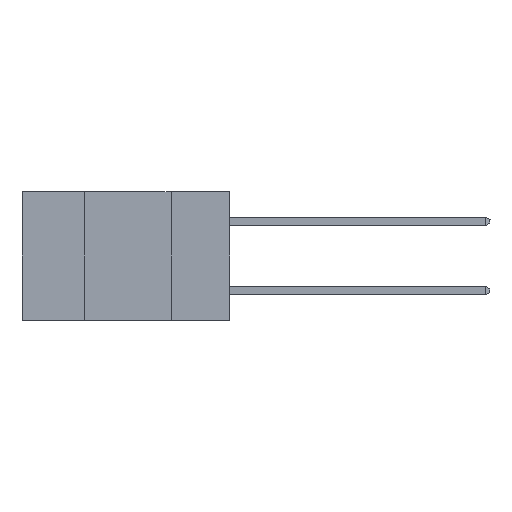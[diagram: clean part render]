
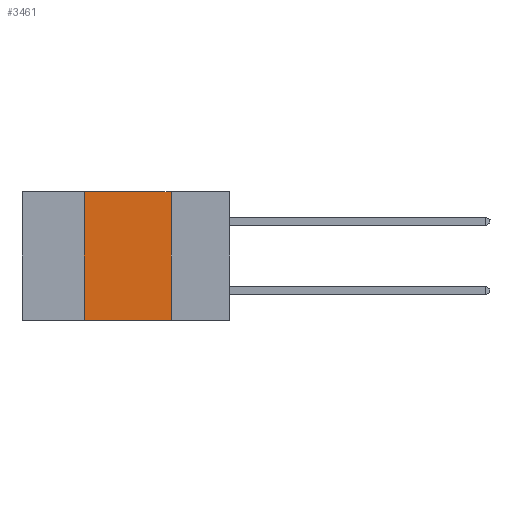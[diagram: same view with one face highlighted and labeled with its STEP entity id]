
A CAD part, left-side view. The second image highlights one B-rep face of the part: STEP entity #3461.
In plain terms, the highlighted planar face has unit normal (-1, 0, 0).
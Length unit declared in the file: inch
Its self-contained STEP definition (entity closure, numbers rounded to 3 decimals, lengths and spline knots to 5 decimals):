
#153 = CARTESIAN_POINT ( 'NONE',  ( 0., 0.17, -0.37 ) ) ;
#271 = DIRECTION ( 'NONE',  ( 0., 0., -1. ) ) ;
#1274 = EDGE_CURVE ( 'NONE', #13791, #14344, #12036, .T. ) ;
#1382 = FACE_OUTER_BOUND ( 'NONE', #9285, .T. ) ;
#2335 = DIRECTION ( 'NONE',  ( 0., -1., 0. ) ) ;
#3461 = ADVANCED_FACE ( 'NONE', ( #1382 ), #6351, .F. ) ;
#3529 = ORIENTED_EDGE ( 'NONE', *, *, #1274, .F. ) ;
#4554 = DIRECTION ( 'NONE',  ( 1., 0., 0. ) ) ;
#6351 = PLANE ( 'NONE',  #21138 ) ;
#7571 = LINE ( 'NONE', #23868, #23378 ) ;
#7751 = EDGE_CURVE ( 'NONE', #14344, #20612, #7571, .T. ) ;
#8056 = LINE ( 'NONE', #14474, #9948 ) ;
#9285 = EDGE_LOOP ( 'NONE', ( #13875, #3529, #11448, #18475 ) ) ;
#9948 = VECTOR ( 'NONE', #12006, 39.37008 ) ;
#10503 = CARTESIAN_POINT ( 'NONE',  ( 0., 0.6, 0. ) ) ;
#11448 = ORIENTED_EDGE ( 'NONE', *, *, #13153, .F. ) ;
#12006 = DIRECTION ( 'NONE',  ( 0., 0., 1. ) ) ;
#12036 = LINE ( 'NONE', #17709, #13574 ) ;
#13153 = EDGE_CURVE ( 'NONE', #13260, #13791, #8056, .T. ) ;
#13260 = VERTEX_POINT ( 'NONE', #22858 ) ;
#13574 = VECTOR ( 'NONE', #19741, 39.37008 ) ;
#13791 = VERTEX_POINT ( 'NONE', #21204 ) ;
#13875 = ORIENTED_EDGE ( 'NONE', *, *, #7751, .F. ) ;
#14344 = VERTEX_POINT ( 'NONE', #19740 ) ;
#14474 = CARTESIAN_POINT ( 'NONE',  ( 0., 0.42, 0. ) ) ;
#17122 = VECTOR ( 'NONE', #2335, 39.37008 ) ;
#17709 = CARTESIAN_POINT ( 'NONE',  ( 0., 0.6, 0. ) ) ;
#17733 = LINE ( 'NONE', #24817, #17122 ) ;
#18475 = ORIENTED_EDGE ( 'NONE', *, *, #24310, .T. ) ;
#19740 = CARTESIAN_POINT ( 'NONE',  ( 0., 0.17, 0. ) ) ;
#19741 = DIRECTION ( 'NONE',  ( 0., -1., 0. ) ) ;
#20612 = VERTEX_POINT ( 'NONE', #153 ) ;
#21138 = AXIS2_PLACEMENT_3D ( 'NONE', #10503, #4554, #271 ) ;
#21204 = CARTESIAN_POINT ( 'NONE',  ( 0., 0.42, 0. ) ) ;
#22858 = CARTESIAN_POINT ( 'NONE',  ( 0., 0.42, -0.37 ) ) ;
#23378 = VECTOR ( 'NONE', #23969, 39.37008 ) ;
#23868 = CARTESIAN_POINT ( 'NONE',  ( 0., 0.17, 0. ) ) ;
#23969 = DIRECTION ( 'NONE',  ( 0., 0., -1. ) ) ;
#24310 = EDGE_CURVE ( 'NONE', #13260, #20612, #17733, .T. ) ;
#24817 = CARTESIAN_POINT ( 'NONE',  ( 0., 0.6, -0.37 ) ) ;
